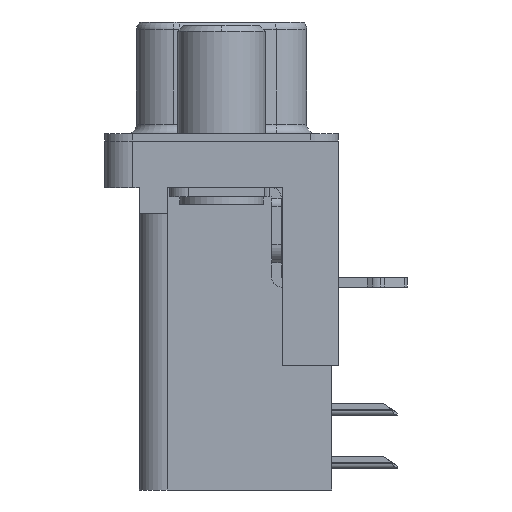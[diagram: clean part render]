
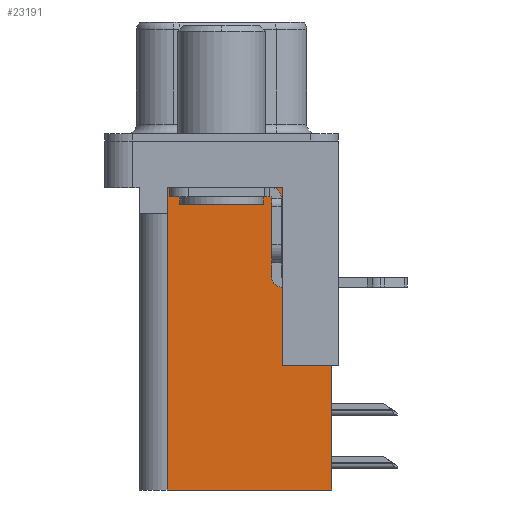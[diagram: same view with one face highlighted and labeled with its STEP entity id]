
A CAD part, left-side view. The second image highlights one B-rep face of the part: STEP entity #23191.
In plain terms, the highlighted planar face has unit normal (-1, 0, 0).
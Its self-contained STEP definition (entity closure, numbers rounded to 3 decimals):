
#358 = LINE ( 'NONE', #21523, #16745 ) ;
#800 = VECTOR ( 'NONE', #25458, 1000. ) ;
#845 = ORIENTED_EDGE ( 'NONE', *, *, #23443, .F. ) ;
#1657 = AXIS2_PLACEMENT_3D ( 'NONE', #26797, #3307, #18243 ) ;
#1696 = LINE ( 'NONE', #6099, #6708 ) ;
#1817 = FACE_OUTER_BOUND ( 'NONE', #16384, .T. ) ;
#3073 = ORIENTED_EDGE ( 'NONE', *, *, #7783, .T. ) ;
#3307 = DIRECTION ( 'NONE',  ( 1., 0., 0. ) ) ;
#3524 = CARTESIAN_POINT ( 'NONE',  ( 3.79, -6.295, -12.05 ) ) ;
#4438 = LINE ( 'NONE', #3524, #20776 ) ;
#4659 = EDGE_CURVE ( 'NONE', #10075, #21039, #358, .T. ) ;
#4720 = CARTESIAN_POINT ( 'NONE',  ( 3.79, 2.925, -3.9 ) ) ;
#4725 = CARTESIAN_POINT ( 'NONE',  ( 3.79, -3.295, -2.5 ) ) ;
#4820 = EDGE_CURVE ( 'NONE', #13924, #10421, #9056, .T. ) ;
#6048 = ORIENTED_EDGE ( 'NONE', *, *, #4659, .F. ) ;
#6099 = CARTESIAN_POINT ( 'NONE',  ( 3.79, 0., -3.9 ) ) ;
#6495 = LINE ( 'NONE', #12613, #800 ) ;
#6650 = CARTESIAN_POINT ( 'NONE',  ( 3.79, 2.895, -3.9 ) ) ;
#6708 = VECTOR ( 'NONE', #8265, 1000. ) ;
#7041 = VECTOR ( 'NONE', #21034, 1000. ) ;
#7783 = EDGE_CURVE ( 'NONE', #16835, #22289, #14306, .T. ) ;
#8265 = DIRECTION ( 'NONE',  ( 0., 1., 0. ) ) ;
#9052 = EDGE_CURVE ( 'NONE', #10421, #16835, #22209, .T. ) ;
#9056 = LINE ( 'NONE', #21220, #7041 ) ;
#9436 = CARTESIAN_POINT ( 'NONE',  ( 3.79, 2.895, -2.5 ) ) ;
#10075 = VERTEX_POINT ( 'NONE', #23263 ) ;
#10421 = VERTEX_POINT ( 'NONE', #22188 ) ;
#10517 = EDGE_CURVE ( 'NONE', #16194, #13924, #4438, .T. ) ;
#10882 = CARTESIAN_POINT ( 'NONE',  ( 3.79, 2.895, -3.9 ) ) ;
#11112 = CARTESIAN_POINT ( 'NONE',  ( 3.79, -5.925, -12.05 ) ) ;
#11154 = CARTESIAN_POINT ( 'NONE',  ( 3.79, -3.295, -12.05 ) ) ;
#12613 = CARTESIAN_POINT ( 'NONE',  ( 3.79, -3.295, -18.76 ) ) ;
#13924 = VERTEX_POINT ( 'NONE', #11154 ) ;
#14155 = ORIENTED_EDGE ( 'NONE', *, *, #10517, .T. ) ;
#14261 = ORIENTED_EDGE ( 'NONE', *, *, #9052, .T. ) ;
#14306 = LINE ( 'NONE', #6650, #25008 ) ;
#16120 = PLANE ( 'NONE',  #1657 ) ;
#16194 = VERTEX_POINT ( 'NONE', #11112 ) ;
#16283 = EDGE_CURVE ( 'NONE', #16194, #17480, #23212, .T. ) ;
#16384 = EDGE_LOOP ( 'NONE', ( #14261, #3073, #24543, #6048, #845, #23600, #14155, #21727 ) ) ;
#16745 = VECTOR ( 'NONE', #18548, 1000. ) ;
#16835 = VERTEX_POINT ( 'NONE', #9436 ) ;
#17480 = VERTEX_POINT ( 'NONE', #24271 ) ;
#17511 = VECTOR ( 'NONE', #22148, 1000. ) ;
#18243 = DIRECTION ( 'NONE',  ( 0., 1., 0. ) ) ;
#18548 = DIRECTION ( 'NONE',  ( 0., 0., 1. ) ) ;
#20776 = VECTOR ( 'NONE', #27091, 1000. ) ;
#21034 = DIRECTION ( 'NONE',  ( 0., 0., 1. ) ) ;
#21039 = VERTEX_POINT ( 'NONE', #4720 ) ;
#21220 = CARTESIAN_POINT ( 'NONE',  ( 3.79, -3.295, -18.76 ) ) ;
#21523 = CARTESIAN_POINT ( 'NONE',  ( 3.79, 2.925, -18.76 ) ) ;
#21528 = VECTOR ( 'NONE', #26230, 1000. ) ;
#21727 = ORIENTED_EDGE ( 'NONE', *, *, #4820, .T. ) ;
#22148 = DIRECTION ( 'NONE',  ( 0., 0., -1. ) ) ;
#22188 = CARTESIAN_POINT ( 'NONE',  ( 3.79, -3.295, -2.5 ) ) ;
#22209 = LINE ( 'NONE', #4725, #21528 ) ;
#22289 = VERTEX_POINT ( 'NONE', #10882 ) ;
#22308 = DIRECTION ( 'NONE',  ( 0., 0., -1. ) ) ;
#23191 = ADVANCED_FACE ( 'NONE', ( #1817 ), #16120, .F. ) ;
#23212 = LINE ( 'NONE', #26403, #17511 ) ;
#23263 = CARTESIAN_POINT ( 'NONE',  ( 3.79, 2.925, -18.76 ) ) ;
#23443 = EDGE_CURVE ( 'NONE', #17480, #10075, #6495, .T. ) ;
#23600 = ORIENTED_EDGE ( 'NONE', *, *, #16283, .F. ) ;
#24271 = CARTESIAN_POINT ( 'NONE',  ( 3.79, -5.925, -18.76 ) ) ;
#24543 = ORIENTED_EDGE ( 'NONE', *, *, #25495, .T. ) ;
#25008 = VECTOR ( 'NONE', #22308, 1000. ) ;
#25458 = DIRECTION ( 'NONE',  ( 0., 1., 0. ) ) ;
#25495 = EDGE_CURVE ( 'NONE', #22289, #21039, #1696, .T. ) ;
#26230 = DIRECTION ( 'NONE',  ( 0., 1., 0. ) ) ;
#26403 = CARTESIAN_POINT ( 'NONE',  ( 3.79, -5.925, -2. ) ) ;
#26797 = CARTESIAN_POINT ( 'NONE',  ( 3.79, -3.295, -18.76 ) ) ;
#27091 = DIRECTION ( 'NONE',  ( 0., 1., 0. ) ) ;
